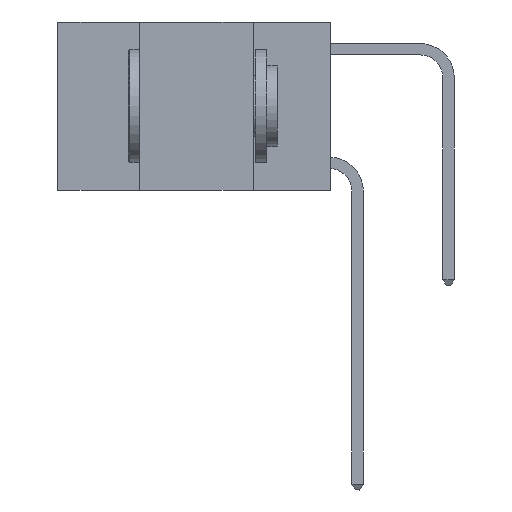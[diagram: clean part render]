
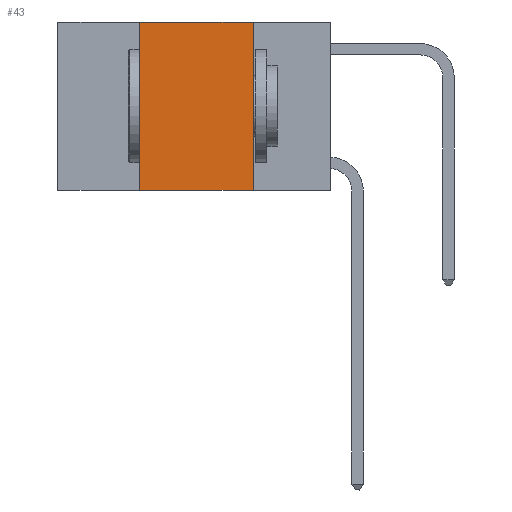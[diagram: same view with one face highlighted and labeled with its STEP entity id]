
A CAD part, left-side view. The second image highlights one B-rep face of the part: STEP entity #43.
In plain terms, the highlighted planar face has unit normal (-1, 0, 0).
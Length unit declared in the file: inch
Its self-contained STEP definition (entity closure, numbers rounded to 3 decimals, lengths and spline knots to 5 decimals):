
#43 = ADVANCED_FACE ( 'NONE', ( #4446 ), #8333, .F. ) ;
#1000 = VERTEX_POINT ( 'NONE', #6518 ) ;
#1358 = DIRECTION ( 'NONE',  ( 0., -1., 0. ) ) ;
#1921 = ORIENTED_EDGE ( 'NONE', *, *, #15156, .T. ) ;
#2125 = ORIENTED_EDGE ( 'NONE', *, *, #16026, .F. ) ;
#2909 = VERTEX_POINT ( 'NONE', #8170 ) ;
#3192 = LINE ( 'NONE', #5593, #9784 ) ;
#3974 = CARTESIAN_POINT ( 'NONE',  ( 0., 0.42, 0. ) ) ;
#4446 = FACE_OUTER_BOUND ( 'NONE', #7540, .T. ) ;
#5367 = DIRECTION ( 'NONE',  ( 0., 0., -1. ) ) ;
#5386 = CARTESIAN_POINT ( 'NONE',  ( 0., 0.6, 0. ) ) ;
#5593 = CARTESIAN_POINT ( 'NONE',  ( 0., 0.42, 0. ) ) ;
#5905 = VECTOR ( 'NONE', #11755, 39.37008 ) ;
#6518 = CARTESIAN_POINT ( 'NONE',  ( 0., 0.17, 0. ) ) ;
#6538 = CARTESIAN_POINT ( 'NONE',  ( 0., 0.6, -0.37 ) ) ;
#7540 = EDGE_LOOP ( 'NONE', ( #8008, #11094, #2125, #1921 ) ) ;
#8008 = ORIENTED_EDGE ( 'NONE', *, *, #16895, .F. ) ;
#8170 = CARTESIAN_POINT ( 'NONE',  ( 0., 0.42, -0.37 ) ) ;
#8333 = PLANE ( 'NONE',  #8670 ) ;
#8670 = AXIS2_PLACEMENT_3D ( 'NONE', #9305, #9781, #15808 ) ;
#9305 = CARTESIAN_POINT ( 'NONE',  ( 0., 0.6, 0. ) ) ;
#9408 = LINE ( 'NONE', #6538, #5905 ) ;
#9457 = DIRECTION ( 'NONE',  ( 0., 0., 1. ) ) ;
#9781 = DIRECTION ( 'NONE',  ( 1., 0., 0. ) ) ;
#9784 = VECTOR ( 'NONE', #9457, 39.37008 ) ;
#9981 = LINE ( 'NONE', #5386, #14688 ) ;
#10004 = VERTEX_POINT ( 'NONE', #3974 ) ;
#11094 = ORIENTED_EDGE ( 'NONE', *, *, #16241, .F. ) ;
#11755 = DIRECTION ( 'NONE',  ( 0., -1., 0. ) ) ;
#13234 = CARTESIAN_POINT ( 'NONE',  ( 0., 0.17, 0. ) ) ;
#13987 = LINE ( 'NONE', #13234, #14388 ) ;
#14388 = VECTOR ( 'NONE', #5367, 39.37008 ) ;
#14502 = VERTEX_POINT ( 'NONE', #15732 ) ;
#14688 = VECTOR ( 'NONE', #1358, 39.37008 ) ;
#15156 = EDGE_CURVE ( 'NONE', #2909, #14502, #9408, .T. ) ;
#15732 = CARTESIAN_POINT ( 'NONE',  ( 0., 0.17, -0.37 ) ) ;
#15808 = DIRECTION ( 'NONE',  ( 0., 0., -1. ) ) ;
#16026 = EDGE_CURVE ( 'NONE', #2909, #10004, #3192, .T. ) ;
#16241 = EDGE_CURVE ( 'NONE', #10004, #1000, #9981, .T. ) ;
#16895 = EDGE_CURVE ( 'NONE', #1000, #14502, #13987, .T. ) ;
